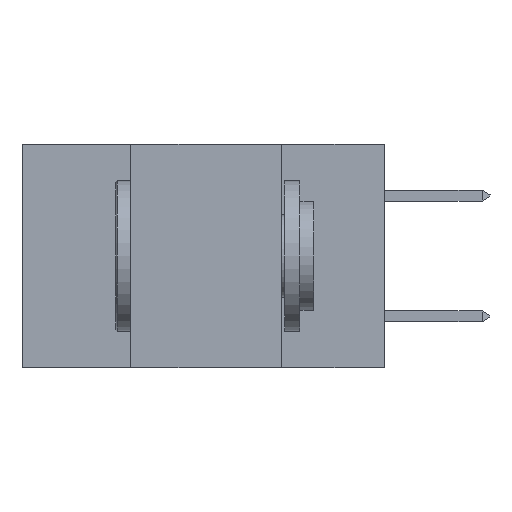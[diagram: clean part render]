
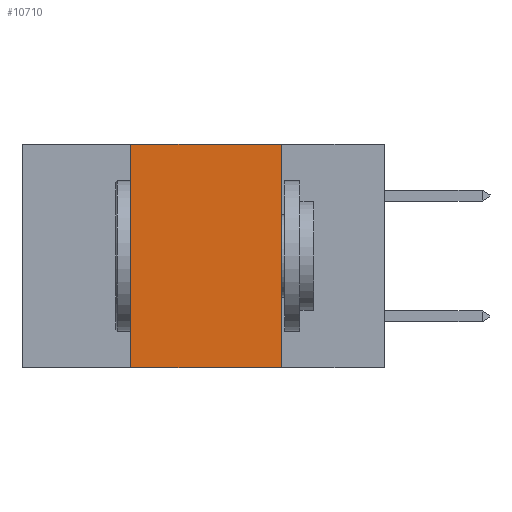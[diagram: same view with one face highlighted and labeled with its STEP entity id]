
A CAD part, left-side view. The second image highlights one B-rep face of the part: STEP entity #10710.
In plain terms, the highlighted planar face has unit normal (-1, 0, 0).
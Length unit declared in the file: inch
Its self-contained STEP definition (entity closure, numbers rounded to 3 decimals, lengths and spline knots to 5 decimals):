
#1809 = CARTESIAN_POINT ( 'NONE',  ( 0., 0.6, 0. ) ) ;
#2211 = PLANE ( 'NONE',  #16580 ) ;
#2515 = ORIENTED_EDGE ( 'NONE', *, *, #30952, .F. ) ;
#4173 = LINE ( 'NONE', #28611, #13215 ) ;
#5134 = DIRECTION ( 'NONE',  ( 0., 0., -1. ) ) ;
#5389 = LINE ( 'NONE', #34031, #18149 ) ;
#6070 = VERTEX_POINT ( 'NONE', #13543 ) ;
#8266 = CARTESIAN_POINT ( 'NONE',  ( 0., 0.42, 0. ) ) ;
#9198 = CARTESIAN_POINT ( 'NONE',  ( 0., 0.17, 0. ) ) ;
#9576 = LINE ( 'NONE', #8266, #24693 ) ;
#10279 = DIRECTION ( 'NONE',  ( 0., -1., 0. ) ) ;
#10710 = ADVANCED_FACE ( 'NONE', ( #13062 ), #2211, .F. ) ;
#10844 = LINE ( 'NONE', #9198, #16971 ) ;
#12684 = CARTESIAN_POINT ( 'NONE',  ( 0., 0.42, -0.37 ) ) ;
#13062 = FACE_OUTER_BOUND ( 'NONE', #29040, .T. ) ;
#13215 = VECTOR ( 'NONE', #31650, 39.37008 ) ;
#13543 = CARTESIAN_POINT ( 'NONE',  ( 0., 0.42, 0. ) ) ;
#13561 = CARTESIAN_POINT ( 'NONE',  ( 0., 0.17, 0. ) ) ;
#13659 = VERTEX_POINT ( 'NONE', #13561 ) ;
#15198 = DIRECTION ( 'NONE',  ( 0., 0., -1. ) ) ;
#16580 = AXIS2_PLACEMENT_3D ( 'NONE', #1809, #30094, #5134 ) ;
#16819 = ORIENTED_EDGE ( 'NONE', *, *, #26488, .F. ) ;
#16971 = VECTOR ( 'NONE', #15198, 39.37008 ) ;
#18149 = VECTOR ( 'NONE', #10279, 39.37008 ) ;
#18510 = ORIENTED_EDGE ( 'NONE', *, *, #26301, .T. ) ;
#20541 = VERTEX_POINT ( 'NONE', #12684 ) ;
#23627 = DIRECTION ( 'NONE',  ( 0., 0., 1. ) ) ;
#24693 = VECTOR ( 'NONE', #23627, 39.37008 ) ;
#26301 = EDGE_CURVE ( 'NONE', #20541, #33366, #4173, .T. ) ;
#26488 = EDGE_CURVE ( 'NONE', #13659, #33366, #10844, .T. ) ;
#27692 = CARTESIAN_POINT ( 'NONE',  ( 0., 0.17, -0.37 ) ) ;
#28611 = CARTESIAN_POINT ( 'NONE',  ( 0., 0.6, -0.37 ) ) ;
#29040 = EDGE_LOOP ( 'NONE', ( #16819, #37147, #2515, #18510 ) ) ;
#30094 = DIRECTION ( 'NONE',  ( 1., 0., 0. ) ) ;
#30622 = EDGE_CURVE ( 'NONE', #6070, #13659, #5389, .T. ) ;
#30952 = EDGE_CURVE ( 'NONE', #20541, #6070, #9576, .T. ) ;
#31650 = DIRECTION ( 'NONE',  ( 0., -1., 0. ) ) ;
#33366 = VERTEX_POINT ( 'NONE', #27692 ) ;
#34031 = CARTESIAN_POINT ( 'NONE',  ( 0., 0.6, 0. ) ) ;
#37147 = ORIENTED_EDGE ( 'NONE', *, *, #30622, .F. ) ;
